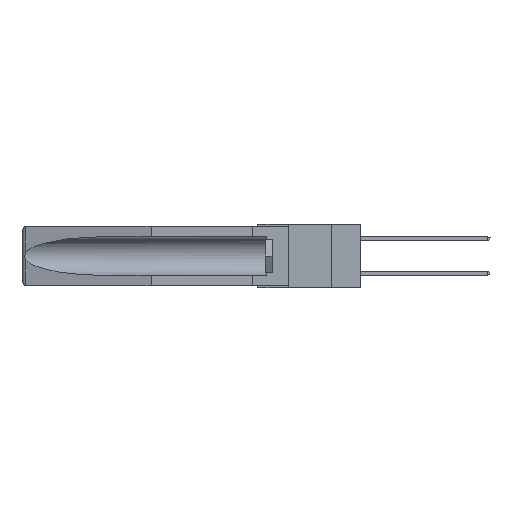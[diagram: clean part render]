
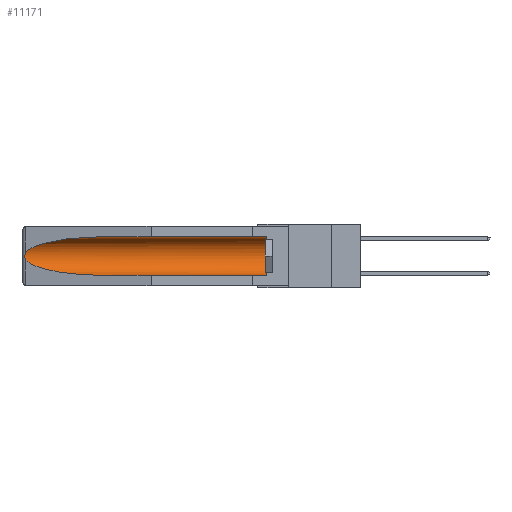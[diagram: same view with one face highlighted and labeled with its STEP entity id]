
A CAD part, left-side view. The second image highlights one B-rep face of the part: STEP entity #11171.
In plain terms, the highlighted cylindrical face has radius 2.857 mm (diameter 5.715 mm), a partial arc.
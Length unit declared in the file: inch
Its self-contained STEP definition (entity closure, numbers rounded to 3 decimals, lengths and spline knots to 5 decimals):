
#58 = CARTESIAN_POINT ( 'NONE',  ( 0.155, 0.126, -0.284 ) ) ;
#159 = CARTESIAN_POINT ( 'NONE',  ( 0.155, 1.07973, -0.059 ) ) ;
#451 = VERTEX_POINT ( 'NONE', #14134 ) ;
#469 = CARTESIAN_POINT ( 'NONE',  ( 0.2673, 1.5327, -0.16383 ) ) ;
#568 = CARTESIAN_POINT ( 'NONE',  ( 0.155, -0.30754, -0.284 ) ) ;
#1882 = DIRECTION ( 'NONE',  ( 0., 0., 1. ) ) ;
#1887 = CARTESIAN_POINT ( 'NONE',  ( 0.25451, 1.48313, -0.09465 ) ) ;
#1915 = CARTESIAN_POINT ( 'NONE',  ( 0.26537, 1.52718, -0.19328 ) ) ;
#2198 = CARTESIAN_POINT ( 'NONE',  ( 0.25451, 1.48313, -0.24835 ) ) ;
#2337 = CARTESIAN_POINT ( 'NONE',  ( 0.26654, 1.53092, -0.15636 ) ) ;
#2364 = CARTESIAN_POINT ( 'NONE',  ( 0.155, 1.07973, -0.284 ) ) ;
#2507 = EDGE_CURVE ( 'NONE', #2560, #21421, #22083, .T. ) ;
#2560 = VERTEX_POINT ( 'NONE', #11190 ) ;
#3544 = DIRECTION ( 'NONE',  ( 0., 1., 0. ) ) ;
#3628 = CARTESIAN_POINT ( 'NONE',  ( 0.26537, 1.52718, -0.19328 ) ) ;
#3715 = EDGE_CURVE ( 'NONE', #15989, #2560, #14067, .T. ) ;
#4008 = CARTESIAN_POINT ( 'NONE',  ( 0.26537, 1.52718, -0.14972 ) ) ;
#4507 = DIRECTION ( 'NONE',  ( 0., -1., 0. ) ) ;
#5266 = EDGE_LOOP ( 'NONE', ( #5922, #7840, #21966, #11080, #7541, #8868 ) ) ;
#5864 = CIRCLE ( 'NONE', #13701, 0.1125 ) ;
#5922 = ORIENTED_EDGE ( 'NONE', *, *, #3715, .T. ) ;
#6004 = CARTESIAN_POINT ( 'NONE',  ( 0.26597, 1.5296, -0.19026 ) ) ;
#6066 =( BOUNDED_CURVE ( )  B_SPLINE_CURVE ( 3, ( #3628, #2198, #10526, #14060 ),
 .UNSPECIFIED., .F., .F. ) 
 B_SPLINE_CURVE_WITH_KNOTS ( ( 4, 4 ),
 ( 0.1948, 1.5708 ),
 .UNSPECIFIED. ) 
 CURVE ( )  GEOMETRIC_REPRESENTATION_ITEM ( )  RATIONAL_B_SPLINE_CURVE ( ( 1., 0.848, 0.848, 1. ) ) 
 REPRESENTATION_ITEM ( '' )  );
#6512 = CARTESIAN_POINT ( 'NONE',  ( 0.155, 1.07973, -0.059 ) ) ;
#6636 = VERTEX_POINT ( 'NONE', #58 ) ;
#7296 = CARTESIAN_POINT ( 'NONE',  ( 0.155, -0.30754, -0.059 ) ) ;
#7541 = ORIENTED_EDGE ( 'NONE', *, *, #17965, .T. ) ;
#7840 = ORIENTED_EDGE ( 'NONE', *, *, #2507, .T. ) ;
#8155 = CARTESIAN_POINT ( 'NONE',  ( 0.155, 0.126, -0.1715 ) ) ;
#8531 = LINE ( 'NONE', #568, #10421 ) ;
#8868 = ORIENTED_EDGE ( 'NONE', *, *, #9109, .T. ) ;
#8874 = EDGE_CURVE ( 'NONE', #21421, #21560, #6066, .T. ) ;
#9109 = EDGE_CURVE ( 'NONE', #451, #15989, #20826, .T. ) ;
#9813 = DIRECTION ( 'NONE',  ( 0., 0., 1. ) ) ;
#9832 = CYLINDRICAL_SURFACE ( 'NONE', #14576, 0.1125 ) ;
#10421 = VECTOR ( 'NONE', #12938, 39.37008 ) ;
#10526 = CARTESIAN_POINT ( 'NONE',  ( 0.21114, 1.30732, -0.284 ) ) ;
#10759 = CARTESIAN_POINT ( 'NONE',  ( 0.2675, 1.53308, -0.16763 ) ) ;
#11080 = ORIENTED_EDGE ( 'NONE', *, *, #21290, .F. ) ;
#11171 = ADVANCED_FACE ( 'NONE', ( #11943 ), #9832, .F. ) ;
#11190 = CARTESIAN_POINT ( 'NONE',  ( 0.26537, 1.52718, -0.14972 ) ) ;
#11943 = FACE_OUTER_BOUND ( 'NONE', #5266, .T. ) ;
#12151 = CARTESIAN_POINT ( 'NONE',  ( 0.21114, 1.30732, -0.059 ) ) ;
#12770 = CARTESIAN_POINT ( 'NONE',  ( 0.2673, 1.53269, -0.17917 ) ) ;
#12938 = DIRECTION ( 'NONE',  ( 0., 1., 0. ) ) ;
#13701 = AXIS2_PLACEMENT_3D ( 'NONE', #8155, #4507, #9813 ) ;
#13751 = DIRECTION ( 'NONE',  ( 0., 1., 0. ) ) ;
#14060 = CARTESIAN_POINT ( 'NONE',  ( 0.155, 1.07973, -0.284 ) ) ;
#14067 =( BOUNDED_CURVE ( )  B_SPLINE_CURVE ( 3, ( #159, #12151, #1887, #18897 ),
 .UNSPECIFIED., .F., .F. ) 
 B_SPLINE_CURVE_WITH_KNOTS ( ( 4, 4 ),
 ( 4.71239, 6.08839 ),
 .UNSPECIFIED. ) 
 CURVE ( )  GEOMETRIC_REPRESENTATION_ITEM ( )  RATIONAL_B_SPLINE_CURVE ( ( 1., 0.848, 0.848, 1. ) ) 
 REPRESENTATION_ITEM ( '' )  );
#14134 = CARTESIAN_POINT ( 'NONE',  ( 0.155, 0.126, -0.059 ) ) ;
#14576 = AXIS2_PLACEMENT_3D ( 'NONE', #15417, #13751, #1882 ) ;
#14584 = CARTESIAN_POINT ( 'NONE',  ( 0.26655, 1.53094, -0.18657 ) ) ;
#15417 = CARTESIAN_POINT ( 'NONE',  ( 0.155, -0.30754, -0.1715 ) ) ;
#15989 = VERTEX_POINT ( 'NONE', #6512 ) ;
#16252 = CARTESIAN_POINT ( 'NONE',  ( 0.26537, 1.52718, -0.19328 ) ) ;
#17341 = VECTOR ( 'NONE', #3544, 39.37008 ) ;
#17965 = EDGE_CURVE ( 'NONE', #6636, #451, #5864, .T. ) ;
#18897 = CARTESIAN_POINT ( 'NONE',  ( 0.26537, 1.52718, -0.14972 ) ) ;
#20826 = LINE ( 'NONE', #7296, #17341 ) ;
#20997 = CARTESIAN_POINT ( 'NONE',  ( 0.26597, 1.52961, -0.15275 ) ) ;
#21290 = EDGE_CURVE ( 'NONE', #6636, #21560, #8531, .T. ) ;
#21421 = VERTEX_POINT ( 'NONE', #1915 ) ;
#21432 = CARTESIAN_POINT ( 'NONE',  ( 0.2675, 1.53308, -0.17534 ) ) ;
#21560 = VERTEX_POINT ( 'NONE', #2364 ) ;
#21966 = ORIENTED_EDGE ( 'NONE', *, *, #8874, .T. ) ;
#22083 = B_SPLINE_CURVE_WITH_KNOTS ( 'NONE', 3,
 ( #4008, #20997, #2337, #469, #10759, #21432, #12770, #14584, #6004, #16252 ),
 .UNSPECIFIED., .F., .F.,
 ( 4, 2, 2, 2, 4 ),
 ( 0., 0.00029, 0.00058, 0.00087, 0.00117 ),
 .UNSPECIFIED. ) ;
